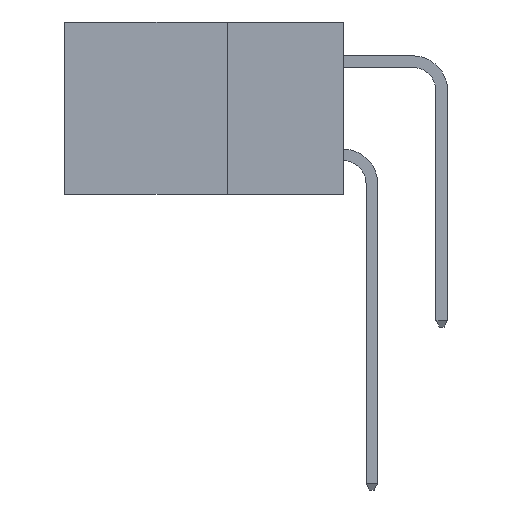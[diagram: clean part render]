
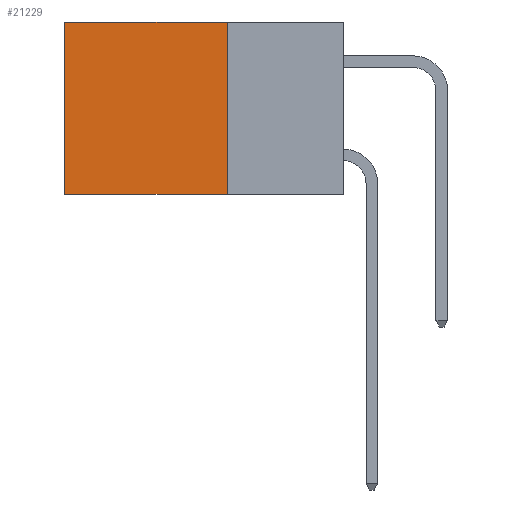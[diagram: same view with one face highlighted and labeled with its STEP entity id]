
A CAD part, left-side view. The second image highlights one B-rep face of the part: STEP entity #21229.
In plain terms, the highlighted planar face has unit normal (-1, 0, 0).
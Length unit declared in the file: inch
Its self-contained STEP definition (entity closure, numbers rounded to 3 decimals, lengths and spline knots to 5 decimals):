
#499 = CARTESIAN_POINT ( 'NONE',  ( 0.2615, 0.6, -0.37 ) ) ;
#1177 = ORIENTED_EDGE ( 'NONE', *, *, #1779, .F. ) ;
#1779 = EDGE_CURVE ( 'NONE', #3720, #3158, #13545, .T. ) ;
#1958 = FACE_OUTER_BOUND ( 'NONE', #16327, .T. ) ;
#3107 = EDGE_CURVE ( 'NONE', #11755, #14683, #21558, .T. ) ;
#3158 = VERTEX_POINT ( 'NONE', #7935 ) ;
#3203 = VECTOR ( 'NONE', #24170, 39.37008 ) ;
#3451 = CARTESIAN_POINT ( 'NONE',  ( 0.2615, 0.6, -0.37 ) ) ;
#3720 = VERTEX_POINT ( 'NONE', #15764 ) ;
#4359 = VECTOR ( 'NONE', #5656, 39.37008 ) ;
#4438 = PLANE ( 'NONE',  #10355 ) ;
#5656 = DIRECTION ( 'NONE',  ( 0., 0., -1. ) ) ;
#5963 = DIRECTION ( 'NONE',  ( 0., 1., 0. ) ) ;
#7402 = ORIENTED_EDGE ( 'NONE', *, *, #12440, .F. ) ;
#7935 = CARTESIAN_POINT ( 'NONE',  ( 0.2615, 0.25, -0.37 ) ) ;
#8049 = VECTOR ( 'NONE', #8177, 39.37008 ) ;
#8177 = DIRECTION ( 'NONE',  ( 0., 0., -1. ) ) ;
#9682 = CARTESIAN_POINT ( 'NONE',  ( 0.2615, 0.25, 0. ) ) ;
#10355 = AXIS2_PLACEMENT_3D ( 'NONE', #23127, #10727, #25196 ) ;
#10727 = DIRECTION ( 'NONE',  ( 1., 0., 0. ) ) ;
#11755 = VERTEX_POINT ( 'NONE', #18129 ) ;
#12440 = EDGE_CURVE ( 'NONE', #3158, #14683, #20029, .T. ) ;
#13545 = LINE ( 'NONE', #26806, #8049 ) ;
#14683 = VERTEX_POINT ( 'NONE', #499 ) ;
#14903 = LINE ( 'NONE', #9682, #3203 ) ;
#15764 = CARTESIAN_POINT ( 'NONE',  ( 0.2615, 0.25, 0. ) ) ;
#16327 = EDGE_LOOP ( 'NONE', ( #19543, #7402, #1177, #23240 ) ) ;
#18129 = CARTESIAN_POINT ( 'NONE',  ( 0.2615, 0.6, 0. ) ) ;
#19543 = ORIENTED_EDGE ( 'NONE', *, *, #3107, .T. ) ;
#20029 = LINE ( 'NONE', #20466, #24898 ) ;
#20466 = CARTESIAN_POINT ( 'NONE',  ( 0.2615, 0.25, -0.37 ) ) ;
#21229 = ADVANCED_FACE ( 'NONE', ( #1958 ), #4438, .F. ) ;
#21558 = LINE ( 'NONE', #3451, #4359 ) ;
#22347 = EDGE_CURVE ( 'NONE', #3720, #11755, #14903, .T. ) ;
#23127 = CARTESIAN_POINT ( 'NONE',  ( 0.2615, 0.25, -0.37 ) ) ;
#23240 = ORIENTED_EDGE ( 'NONE', *, *, #22347, .T. ) ;
#24170 = DIRECTION ( 'NONE',  ( 0., 1., 0. ) ) ;
#24898 = VECTOR ( 'NONE', #5963, 39.37008 ) ;
#25196 = DIRECTION ( 'NONE',  ( 0., 0., -1. ) ) ;
#26806 = CARTESIAN_POINT ( 'NONE',  ( 0.2615, 0.25, -0.37 ) ) ;
